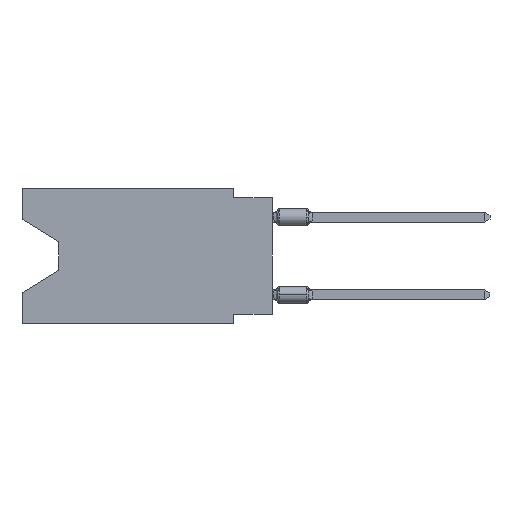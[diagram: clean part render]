
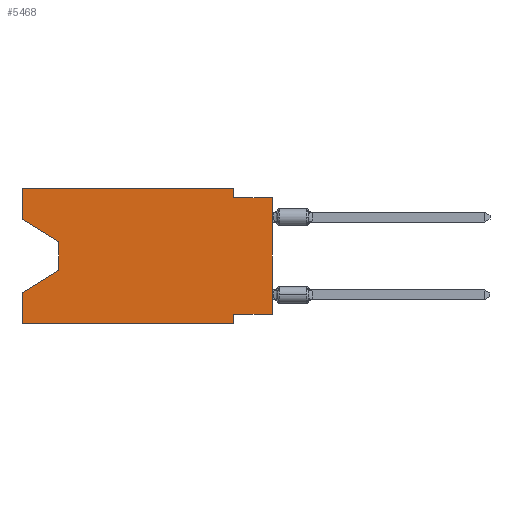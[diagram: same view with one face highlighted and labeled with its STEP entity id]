
A CAD part, left-side view. The second image highlights one B-rep face of the part: STEP entity #5468.
In plain terms, the highlighted planar face has unit normal (-1, 0, 0).
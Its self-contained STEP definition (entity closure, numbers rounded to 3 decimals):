
#102 = VERTEX_POINT ( 'NONE', #3472 ) ;
#108 = VECTOR ( 'NONE', #1853, 1000. ) ;
#232 = ORIENTED_EDGE ( 'NONE', *, *, #7577, .T. ) ;
#304 = VERTEX_POINT ( 'NONE', #4538 ) ;
#572 = ORIENTED_EDGE ( 'NONE', *, *, #11953, .F. ) ;
#1041 = CARTESIAN_POINT ( 'NONE',  ( 0., 16.383, -2.038 ) ) ;
#1234 = VERTEX_POINT ( 'NONE', #8981 ) ;
#1437 = VERTEX_POINT ( 'NONE', #5194 ) ;
#1739 = DIRECTION ( 'NONE',  ( 0., 0., 1. ) ) ;
#1846 = LINE ( 'NONE', #6114, #8120 ) ;
#1853 = DIRECTION ( 'NONE',  ( 0., 0., -1. ) ) ;
#1912 = CARTESIAN_POINT ( 'NONE',  ( 0., 2.54, -0.635 ) ) ;
#1917 = VERTEX_POINT ( 'NONE', #13472 ) ;
#1962 = VECTOR ( 'NONE', #13602, 1000. ) ;
#2179 = VECTOR ( 'NONE', #3022, 1000. ) ;
#2247 = CARTESIAN_POINT ( 'NONE',  ( 0., 13.97, -3.505 ) ) ;
#2263 = CARTESIAN_POINT ( 'NONE',  ( 0., 16.383, 0. ) ) ;
#3022 = DIRECTION ( 'NONE',  ( 0., 0., -1. ) ) ;
#3051 = CARTESIAN_POINT ( 'NONE',  ( 0., 0., -8.255 ) ) ;
#3241 = ORIENTED_EDGE ( 'NONE', *, *, #11052, .F. ) ;
#3472 = CARTESIAN_POINT ( 'NONE',  ( 0., 16.383, -8.89 ) ) ;
#3633 = VECTOR ( 'NONE', #4738, 1000. ) ;
#3758 = ORIENTED_EDGE ( 'NONE', *, *, #7530, .T. ) ;
#3801 = CARTESIAN_POINT ( 'NONE',  ( 0., 16.383, 0. ) ) ;
#3865 = VERTEX_POINT ( 'NONE', #6283 ) ;
#3940 = VECTOR ( 'NONE', #11155, 1000. ) ;
#3957 = DIRECTION ( 'NONE',  ( 0., 0., 1. ) ) ;
#4212 = PLANE ( 'NONE',  #7238 ) ;
#4538 = CARTESIAN_POINT ( 'NONE',  ( 0., 16.383, -2.038 ) ) ;
#4596 = ORIENTED_EDGE ( 'NONE', *, *, #12776, .T. ) ;
#4738 = DIRECTION ( 'NONE',  ( 0., -1., 0. ) ) ;
#4909 = LINE ( 'NONE', #3801, #13186 ) ;
#4981 = CARTESIAN_POINT ( 'NONE',  ( 0., 0., -8.255 ) ) ;
#5159 = CARTESIAN_POINT ( 'NONE',  ( 0., 2.54, -8.89 ) ) ;
#5186 = LINE ( 'NONE', #3051, #1962 ) ;
#5194 = CARTESIAN_POINT ( 'NONE',  ( 0., 2.54, -8.89 ) ) ;
#5237 = FACE_OUTER_BOUND ( 'NONE', #13633, .T. ) ;
#5252 = DIRECTION ( 'NONE',  ( 0., -0.855, -0.519 ) ) ;
#5312 = CARTESIAN_POINT ( 'NONE',  ( 0., 16.383, 0. ) ) ;
#5468 = ADVANCED_FACE ( 'NONE', ( #5237 ), #4212, .F. ) ;
#5516 = LINE ( 'NONE', #1041, #13178 ) ;
#5733 = LINE ( 'NONE', #5159, #108 ) ;
#5813 = EDGE_CURVE ( 'NONE', #9185, #12493, #6523, .T. ) ;
#5835 = LINE ( 'NONE', #11908, #9580 ) ;
#5876 = CARTESIAN_POINT ( 'NONE',  ( 0., 0., 0. ) ) ;
#6049 = DIRECTION ( 'NONE',  ( 0., 0., 1. ) ) ;
#6114 = CARTESIAN_POINT ( 'NONE',  ( 0., 16.383, 0. ) ) ;
#6154 = CARTESIAN_POINT ( 'NONE',  ( 0., 13.97, -5.385 ) ) ;
#6283 = CARTESIAN_POINT ( 'NONE',  ( 0., 0., -0.635 ) ) ;
#6523 = LINE ( 'NONE', #2263, #10763 ) ;
#6598 = EDGE_CURVE ( 'NONE', #1234, #7073, #13565, .T. ) ;
#6634 = ORIENTED_EDGE ( 'NONE', *, *, #11925, .F. ) ;
#6860 = ORIENTED_EDGE ( 'NONE', *, *, #6598, .T. ) ;
#6869 = CARTESIAN_POINT ( 'NONE',  ( 0., 16.383, -8.89 ) ) ;
#7073 = VERTEX_POINT ( 'NONE', #6154 ) ;
#7157 = VERTEX_POINT ( 'NONE', #10838 ) ;
#7238 = AXIS2_PLACEMENT_3D ( 'NONE', #5312, #9511, #12830 ) ;
#7281 = EDGE_CURVE ( 'NONE', #7157, #1437, #5733, .T. ) ;
#7530 = EDGE_CURVE ( 'NONE', #7073, #1917, #5835, .T. ) ;
#7577 = EDGE_CURVE ( 'NONE', #102, #1437, #9975, .T. ) ;
#7976 = CARTESIAN_POINT ( 'NONE',  ( 0., 0., -0.635 ) ) ;
#8120 = VECTOR ( 'NONE', #6049, 1000. ) ;
#8415 = ORIENTED_EDGE ( 'NONE', *, *, #5813, .F. ) ;
#8439 = CARTESIAN_POINT ( 'NONE',  ( 0., 2.54, 0. ) ) ;
#8796 = DIRECTION ( 'NONE',  ( 0., 0.855, -0.519 ) ) ;
#8981 = CARTESIAN_POINT ( 'NONE',  ( 0., 13.97, -3.505 ) ) ;
#9084 = ORIENTED_EDGE ( 'NONE', *, *, #9641, .F. ) ;
#9185 = VERTEX_POINT ( 'NONE', #9817 ) ;
#9292 = LINE ( 'NONE', #13513, #2179 ) ;
#9511 = DIRECTION ( 'NONE',  ( 1., 0., 0. ) ) ;
#9580 = VECTOR ( 'NONE', #8796, 1000. ) ;
#9641 = EDGE_CURVE ( 'NONE', #304, #9185, #4909, .T. ) ;
#9817 = CARTESIAN_POINT ( 'NONE',  ( 0., 16.383, 0. ) ) ;
#9975 = LINE ( 'NONE', #6869, #3633 ) ;
#10267 = LINE ( 'NONE', #7976, #3940 ) ;
#10491 = ORIENTED_EDGE ( 'NONE', *, *, #11889, .F. ) ;
#10521 = DIRECTION ( 'NONE',  ( 0., 0., -1. ) ) ;
#10763 = VECTOR ( 'NONE', #11769, 1000. ) ;
#10838 = CARTESIAN_POINT ( 'NONE',  ( 0., 2.54, -8.255 ) ) ;
#11052 = EDGE_CURVE ( 'NONE', #11076, #7157, #5186, .T. ) ;
#11076 = VERTEX_POINT ( 'NONE', #4981 ) ;
#11120 = LINE ( 'NONE', #5876, #12769 ) ;
#11155 = DIRECTION ( 'NONE',  ( 0., -1., 0. ) ) ;
#11208 = EDGE_CURVE ( 'NONE', #304, #1234, #5516, .T. ) ;
#11769 = DIRECTION ( 'NONE',  ( 0., -1., 0. ) ) ;
#11888 = VERTEX_POINT ( 'NONE', #1912 ) ;
#11889 = EDGE_CURVE ( 'NONE', #11888, #3865, #10267, .T. ) ;
#11908 = CARTESIAN_POINT ( 'NONE',  ( 0., 13.97, -5.385 ) ) ;
#11925 = EDGE_CURVE ( 'NONE', #102, #1917, #1846, .T. ) ;
#11953 = EDGE_CURVE ( 'NONE', #12493, #11888, #9292, .T. ) ;
#12493 = VERTEX_POINT ( 'NONE', #8439 ) ;
#12769 = VECTOR ( 'NONE', #3957, 1000. ) ;
#12776 = EDGE_CURVE ( 'NONE', #11076, #3865, #11120, .T. ) ;
#12830 = DIRECTION ( 'NONE',  ( 0., 0., -1. ) ) ;
#13043 = ORIENTED_EDGE ( 'NONE', *, *, #11208, .T. ) ;
#13073 = ORIENTED_EDGE ( 'NONE', *, *, #7281, .F. ) ;
#13178 = VECTOR ( 'NONE', #5252, 1000. ) ;
#13184 = VECTOR ( 'NONE', #10521, 1000. ) ;
#13186 = VECTOR ( 'NONE', #1739, 1000. ) ;
#13472 = CARTESIAN_POINT ( 'NONE',  ( 0., 16.383, -6.852 ) ) ;
#13513 = CARTESIAN_POINT ( 'NONE',  ( 0., 2.54, 0. ) ) ;
#13565 = LINE ( 'NONE', #2247, #13184 ) ;
#13602 = DIRECTION ( 'NONE',  ( 0., 1., 0. ) ) ;
#13633 = EDGE_LOOP ( 'NONE', ( #13043, #6860, #3758, #6634, #232, #13073, #3241, #4596, #10491, #572, #8415, #9084 ) ) ;
